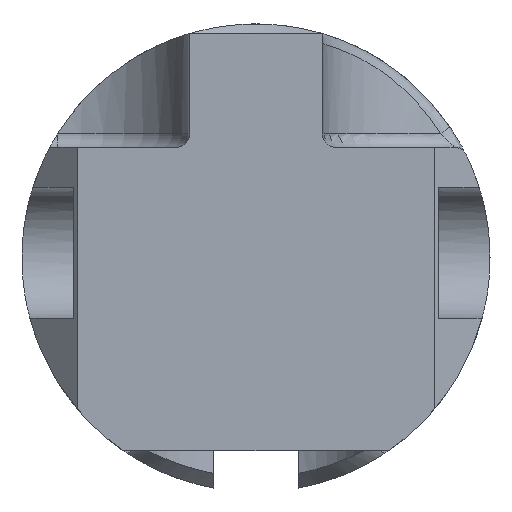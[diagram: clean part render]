
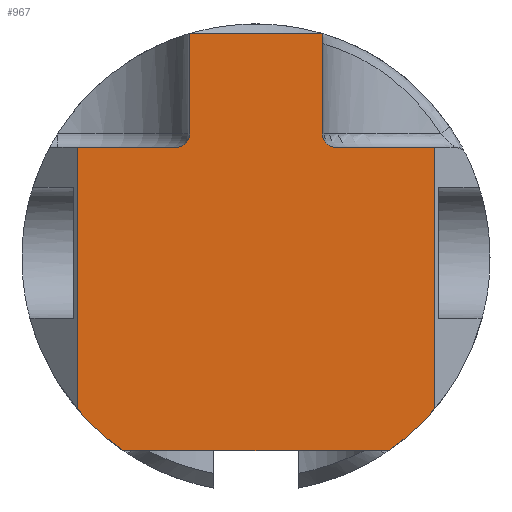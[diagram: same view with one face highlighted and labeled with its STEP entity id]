
A CAD part, front view. The second image highlights one B-rep face of the part: STEP entity #967.
In plain terms, the highlighted planar face has unit normal (0, -1, 0).
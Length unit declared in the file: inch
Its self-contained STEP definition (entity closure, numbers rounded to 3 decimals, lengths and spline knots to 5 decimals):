
#49=CIRCLE('',#1013,0.4375);
#50=CIRCLE('',#1018,0.4375);
#57=CIRCLE('',#1046,0.025);
#58=CIRCLE('',#1047,0.025);
#100=FACE_OUTER_BOUND('',#152,.T.);
#152=EDGE_LOOP('',(#811,#812,#813,#814,#815,#816,#817,#818,#819,#820,#821,
#822));
#222=LINE('',#2111,#299);
#229=LINE('',#2125,#306);
#233=LINE('',#2132,#310);
#234=LINE('',#2134,#311);
#235=LINE('',#2138,#312);
#236=LINE('',#2140,#313);
#237=LINE('',#2142,#314);
#238=LINE('',#2145,#315);
#299=VECTOR('',#1205,0.3937);
#306=VECTOR('',#1216,0.3937);
#310=VECTOR('',#1226,0.3937);
#311=VECTOR('',#1227,0.3937);
#312=VECTOR('',#1230,0.3937);
#313=VECTOR('',#1231,0.3937);
#314=VECTOR('',#1232,0.3937);
#315=VECTOR('',#1235,0.3937);
#388=VERTEX_POINT('',#1423);
#389=VERTEX_POINT('',#1425);
#416=VERTEX_POINT('',#1585);
#417=VERTEX_POINT('',#1587);
#443=VERTEX_POINT('',#2110);
#448=VERTEX_POINT('',#2123);
#449=VERTEX_POINT('',#2133);
#450=VERTEX_POINT('',#2135);
#451=VERTEX_POINT('',#2137);
#452=VERTEX_POINT('',#2139);
#453=VERTEX_POINT('',#2141);
#454=VERTEX_POINT('',#2143);
#490=EDGE_CURVE('',#388,#389,#49,.T.);
#518=EDGE_CURVE('',#416,#417,#50,.T.);
#567=EDGE_CURVE('',#443,#389,#222,.T.);
#575=EDGE_CURVE('',#416,#448,#229,.T.);
#579=EDGE_CURVE('',#388,#417,#233,.T.);
#580=EDGE_CURVE('',#448,#449,#234,.T.);
#581=EDGE_CURVE('',#450,#449,#57,.T.);
#582=EDGE_CURVE('',#450,#451,#235,.T.);
#583=EDGE_CURVE('',#452,#451,#236,.T.);
#584=EDGE_CURVE('',#452,#453,#237,.T.);
#585=EDGE_CURVE('',#454,#453,#58,.T.);
#586=EDGE_CURVE('',#454,#443,#238,.T.);
#811=ORIENTED_EDGE('',*,*,#567,.T.);
#812=ORIENTED_EDGE('',*,*,#490,.F.);
#813=ORIENTED_EDGE('',*,*,#579,.T.);
#814=ORIENTED_EDGE('',*,*,#518,.F.);
#815=ORIENTED_EDGE('',*,*,#575,.T.);
#816=ORIENTED_EDGE('',*,*,#580,.T.);
#817=ORIENTED_EDGE('',*,*,#581,.F.);
#818=ORIENTED_EDGE('',*,*,#582,.T.);
#819=ORIENTED_EDGE('',*,*,#583,.F.);
#820=ORIENTED_EDGE('',*,*,#584,.T.);
#821=ORIENTED_EDGE('',*,*,#585,.F.);
#822=ORIENTED_EDGE('',*,*,#586,.T.);
#925=PLANE('',#1045);
#967=ADVANCED_FACE('',(#100),#925,.F.);
#1013=AXIS2_PLACEMENT_3D('',#1426,#1113,#1114);
#1018=AXIS2_PLACEMENT_3D('',#1588,#1133,#1134);
#1045=AXIS2_PLACEMENT_3D('',#2131,#1224,#1225);
#1046=AXIS2_PLACEMENT_3D('',#2136,#1228,#1229);
#1047=AXIS2_PLACEMENT_3D('',#2144,#1233,#1234);
#1113=DIRECTION('center_axis',(0.,1.,0.));
#1114=DIRECTION('ref_axis',(1.,0.,0.));
#1133=DIRECTION('center_axis',(0.,1.,0.));
#1134=DIRECTION('ref_axis',(1.,0.,0.));
#1205=DIRECTION('',(0.,0.,-1.));
#1216=DIRECTION('',(0.,0.,1.));
#1224=DIRECTION('center_axis',(0.,1.,0.));
#1225=DIRECTION('ref_axis',(1.,0.,0.));
#1226=DIRECTION('',(1.,0.,0.));
#1227=DIRECTION('',(-1.,0.,0.));
#1228=DIRECTION('center_axis',(0.,-1.,0.));
#1229=DIRECTION('ref_axis',(-0.707,0.,-0.707));
#1230=DIRECTION('',(0.,0.,1.));
#1231=DIRECTION('',(1.,0.,0.));
#1232=DIRECTION('',(0.,0.,-1.));
#1233=DIRECTION('center_axis',(0.,-1.,0.));
#1234=DIRECTION('ref_axis',(0.707,0.,-0.707));
#1235=DIRECTION('',(-1.,0.,0.));
#1423=CARTESIAN_POINT('',(-0.2475,0.,-0.36076));
#1425=CARTESIAN_POINT('',(-0.3342,0.,-0.28235));
#1426=CARTESIAN_POINT('Origin',(0.,0.,0.));
#1585=CARTESIAN_POINT('',(0.3342,0.,-0.28235));
#1587=CARTESIAN_POINT('',(0.2475,0.,-0.36076));
#1588=CARTESIAN_POINT('Origin',(0.,0.,0.));
#2110=CARTESIAN_POINT('',(-0.3342,0.,0.20674));
#2111=CARTESIAN_POINT('',(-0.3342,0.,0.0147));
#2123=CARTESIAN_POINT('',(0.3342,0.,0.20674));
#2125=CARTESIAN_POINT('',(0.3342,0.,0.0147));
#2131=CARTESIAN_POINT('Origin',(0.,0.,0.0294));
#2132=CARTESIAN_POINT('',(0.,0.,-0.36076));
#2133=CARTESIAN_POINT('',(0.149,0.,0.20674));
#2134=CARTESIAN_POINT('',(0.19279,0.,0.20674));
#2135=CARTESIAN_POINT('',(0.124,0.,0.23174));
#2136=CARTESIAN_POINT('Origin',(0.149,0.,0.23174));
#2137=CARTESIAN_POINT('',(0.124,0.,0.41956));
#2138=CARTESIAN_POINT('',(0.124,0.,0.11807));
#2139=CARTESIAN_POINT('',(-0.124,0.,0.41956));
#2140=CARTESIAN_POINT('',(-0.124,0.,0.41956));
#2141=CARTESIAN_POINT('',(-0.124,0.,0.23174));
#2142=CARTESIAN_POINT('',(-0.124,0.,0.22448));
#2143=CARTESIAN_POINT('',(-0.149,0.,0.20674));
#2144=CARTESIAN_POINT('Origin',(-0.149,0.,0.23174));
#2145=CARTESIAN_POINT('',(-0.062,0.,0.20674));
